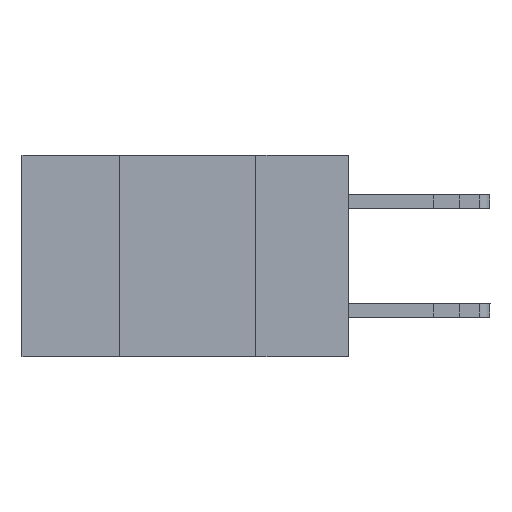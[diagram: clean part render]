
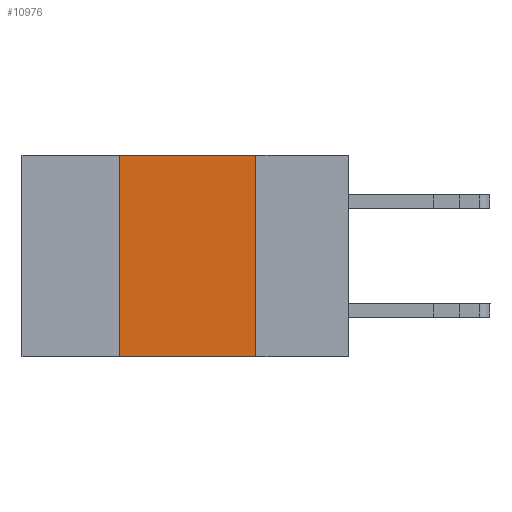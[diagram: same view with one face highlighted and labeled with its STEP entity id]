
A CAD part, left-side view. The second image highlights one B-rep face of the part: STEP entity #10976.
In plain terms, the highlighted planar face has unit normal (-1, 0, 0).
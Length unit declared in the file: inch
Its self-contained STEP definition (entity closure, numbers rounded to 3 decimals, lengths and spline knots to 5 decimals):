
#177 = ORIENTED_EDGE ( 'NONE', *, *, #15688, .F. ) ;
#501 = VERTEX_POINT ( 'NONE', #9506 ) ;
#888 = DIRECTION ( 'NONE',  ( 1., 0., 0. ) ) ;
#1088 = CARTESIAN_POINT ( 'NONE',  ( 0., 0.17, -0.37 ) ) ;
#1325 = EDGE_CURVE ( 'NONE', #13360, #14666, #9673, .T. ) ;
#1584 = ORIENTED_EDGE ( 'NONE', *, *, #12096, .F. ) ;
#1585 = FACE_OUTER_BOUND ( 'NONE', #8188, .T. ) ;
#1871 = CARTESIAN_POINT ( 'NONE',  ( 0., 0.42, 0. ) ) ;
#2506 = DIRECTION ( 'NONE',  ( 0., -1., 0. ) ) ;
#2642 = DIRECTION ( 'NONE',  ( 0., 0., 1. ) ) ;
#3098 = CARTESIAN_POINT ( 'NONE',  ( 0., 0.6, -0.37 ) ) ;
#3394 = CARTESIAN_POINT ( 'NONE',  ( 0., 0.6, 0. ) ) ;
#3437 = LINE ( 'NONE', #3098, #10922 ) ;
#4610 = ORIENTED_EDGE ( 'NONE', *, *, #1325, .F. ) ;
#6229 = LINE ( 'NONE', #14013, #17728 ) ;
#7615 = AXIS2_PLACEMENT_3D ( 'NONE', #12807, #888, #11346 ) ;
#8188 = EDGE_LOOP ( 'NONE', ( #1584, #4610, #177, #11166 ) ) ;
#9506 = CARTESIAN_POINT ( 'NONE',  ( 0., 0.42, -0.37 ) ) ;
#9673 = LINE ( 'NONE', #3394, #13678 ) ;
#9828 = PLANE ( 'NONE',  #7615 ) ;
#10625 = LINE ( 'NONE', #11607, #14151 ) ;
#10922 = VECTOR ( 'NONE', #16611, 39.37008 ) ;
#10976 = ADVANCED_FACE ( 'NONE', ( #1585 ), #9828, .F. ) ;
#11166 = ORIENTED_EDGE ( 'NONE', *, *, #11335, .T. ) ;
#11335 = EDGE_CURVE ( 'NONE', #501, #17618, #3437, .T. ) ;
#11346 = DIRECTION ( 'NONE',  ( 0., 0., -1. ) ) ;
#11607 = CARTESIAN_POINT ( 'NONE',  ( 0., 0.42, -0.37 ) ) ;
#12096 = EDGE_CURVE ( 'NONE', #14666, #17618, #6229, .T. ) ;
#12583 = DIRECTION ( 'NONE',  ( 0., 0., -1. ) ) ;
#12807 = CARTESIAN_POINT ( 'NONE',  ( 0., 0.6, 0. ) ) ;
#13360 = VERTEX_POINT ( 'NONE', #1871 ) ;
#13678 = VECTOR ( 'NONE', #2506, 39.37008 ) ;
#13861 = CARTESIAN_POINT ( 'NONE',  ( 0., 0.17, 0. ) ) ;
#14013 = CARTESIAN_POINT ( 'NONE',  ( 0., 0.17, -0.37 ) ) ;
#14151 = VECTOR ( 'NONE', #2642, 39.37008 ) ;
#14666 = VERTEX_POINT ( 'NONE', #13861 ) ;
#15688 = EDGE_CURVE ( 'NONE', #501, #13360, #10625, .T. ) ;
#16611 = DIRECTION ( 'NONE',  ( 0., -1., 0. ) ) ;
#17618 = VERTEX_POINT ( 'NONE', #1088 ) ;
#17728 = VECTOR ( 'NONE', #12583, 39.37008 ) ;
